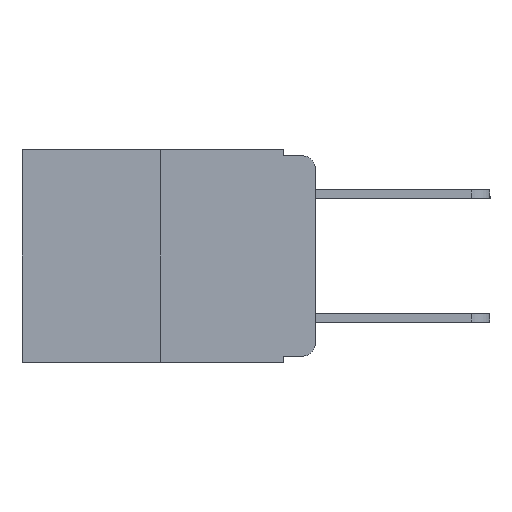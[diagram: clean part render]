
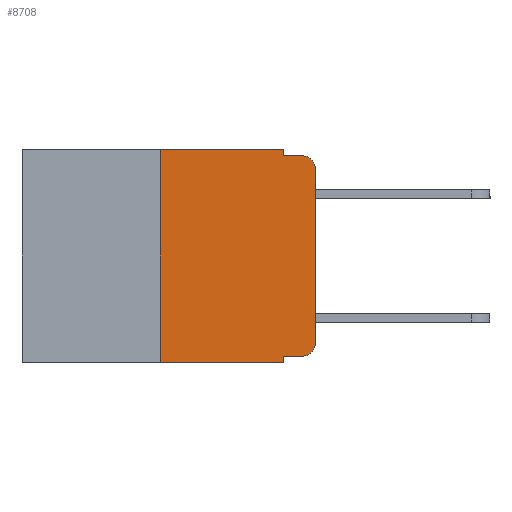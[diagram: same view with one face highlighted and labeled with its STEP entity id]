
A CAD part, left-side view. The second image highlights one B-rep face of the part: STEP entity #8708.
In plain terms, the highlighted planar face has unit normal (-1, 0, 0).
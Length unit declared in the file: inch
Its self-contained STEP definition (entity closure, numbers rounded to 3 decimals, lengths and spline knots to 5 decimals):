
#329 = ORIENTED_EDGE ( 'NONE', *, *, #9230, .F. ) ;
#381 = ORIENTED_EDGE ( 'NONE', *, *, #10804, .T. ) ;
#391 = ORIENTED_EDGE ( 'NONE', *, *, #2260, .F. ) ;
#1883 = CARTESIAN_POINT ( 'NONE',  ( 0., 0.051, -0.01 ) ) ;
#2018 = AXIS2_PLACEMENT_3D ( 'NONE', #16356, #8391, #11238 ) ;
#2258 = DIRECTION ( 'NONE',  ( 0., 0., 1. ) ) ;
#2260 = EDGE_CURVE ( 'NONE', #4453, #10729, #8984, .T. ) ;
#2508 = VERTEX_POINT ( 'NONE', #9882 ) ;
#2665 = CARTESIAN_POINT ( 'NONE',  ( 0., 0.02, -0.313 ) ) ;
#2958 = VECTOR ( 'NONE', #15019, 39.37008 ) ;
#3173 = CARTESIAN_POINT ( 'NONE',  ( 0., 0.051, 0. ) ) ;
#3475 = CARTESIAN_POINT ( 'NONE',  ( 0., 0.02, -0.01 ) ) ;
#3647 = VERTEX_POINT ( 'NONE', #17110 ) ;
#4095 = DIRECTION ( 'NONE',  ( 0., 0., 1. ) ) ;
#4104 = VECTOR ( 'NONE', #10636, 39.37008 ) ;
#4248 = VERTEX_POINT ( 'NONE', #4349 ) ;
#4349 = CARTESIAN_POINT ( 'NONE',  ( 0., 0.25, 0. ) ) ;
#4357 = DIRECTION ( 'NONE',  ( 0., 0., -1. ) ) ;
#4453 = VERTEX_POINT ( 'NONE', #7680 ) ;
#4612 = VERTEX_POINT ( 'NONE', #3475 ) ;
#4946 = LINE ( 'NONE', #14406, #8541 ) ;
#5039 = EDGE_LOOP ( 'NONE', ( #12263, #12685, #16614, #391, #329, #8214, #17254, #11268, #15150, #381 ) ) ;
#5049 = CARTESIAN_POINT ( 'NONE',  ( 0., 0.25, -0.343 ) ) ;
#5187 = VECTOR ( 'NONE', #15256, 39.37008 ) ;
#5480 = CARTESIAN_POINT ( 'NONE',  ( 0., 0.473, -0.343 ) ) ;
#5795 = EDGE_CURVE ( 'NONE', #2508, #3647, #15393, .T. ) ;
#5852 = VECTOR ( 'NONE', #11957, 39.37008 ) ;
#6026 = CARTESIAN_POINT ( 'NONE',  ( 0., 0.051, -0.333 ) ) ;
#7145 = LINE ( 'NONE', #1883, #2958 ) ;
#7378 = PLANE ( 'NONE',  #13105 ) ;
#7387 = EDGE_CURVE ( 'NONE', #15232, #4612, #9110, .T. ) ;
#7433 = CARTESIAN_POINT ( 'NONE',  ( 0., 0.473, 0. ) ) ;
#7680 = CARTESIAN_POINT ( 'NONE',  ( 0., 0.051, 0. ) ) ;
#7707 = LINE ( 'NONE', #3173, #8732 ) ;
#8214 = ORIENTED_EDGE ( 'NONE', *, *, #12314, .F. ) ;
#8391 = DIRECTION ( 'NONE',  ( -1., 0., 0. ) ) ;
#8541 = VECTOR ( 'NONE', #18064, 39.37008 ) ;
#8708 = ADVANCED_FACE ( 'NONE', ( #9063 ), #7378, .F. ) ;
#8732 = VECTOR ( 'NONE', #14728, 39.37008 ) ;
#8843 = VERTEX_POINT ( 'NONE', #17114 ) ;
#8913 = VECTOR ( 'NONE', #4095, 39.37008 ) ;
#8984 = LINE ( 'NONE', #11843, #5852 ) ;
#9034 = DIRECTION ( 'NONE',  ( 0., 0., -1. ) ) ;
#9063 = FACE_OUTER_BOUND ( 'NONE', #5039, .T. ) ;
#9110 = CIRCLE ( 'NONE', #2018, 0.02 ) ;
#9230 = EDGE_CURVE ( 'NONE', #4248, #4453, #4946, .T. ) ;
#9335 = LINE ( 'NONE', #11478, #8913 ) ;
#9690 = CARTESIAN_POINT ( 'NONE',  ( 0., 0.051, -0.343 ) ) ;
#9776 = LINE ( 'NONE', #11377, #16689 ) ;
#9882 = CARTESIAN_POINT ( 'NONE',  ( 0., 0.051, -0.333 ) ) ;
#10411 = VERTEX_POINT ( 'NONE', #5049 ) ;
#10636 = DIRECTION ( 'NONE',  ( 0., -1., 0. ) ) ;
#10729 = VERTEX_POINT ( 'NONE', #11518 ) ;
#10804 = EDGE_CURVE ( 'NONE', #3647, #8843, #18512, .T. ) ;
#11099 = EDGE_CURVE ( 'NONE', #2508, #16935, #7707, .T. ) ;
#11132 = AXIS2_PLACEMENT_3D ( 'NONE', #2665, #13030, #4357 ) ;
#11238 = DIRECTION ( 'NONE',  ( 0., 0., -1. ) ) ;
#11268 = ORIENTED_EDGE ( 'NONE', *, *, #11099, .F. ) ;
#11377 = CARTESIAN_POINT ( 'NONE',  ( 0., 0., 0. ) ) ;
#11478 = CARTESIAN_POINT ( 'NONE',  ( 0., 0.25, 0. ) ) ;
#11518 = CARTESIAN_POINT ( 'NONE',  ( 0., 0.051, -0.01 ) ) ;
#11843 = CARTESIAN_POINT ( 'NONE',  ( 0., 0.051, 0. ) ) ;
#11957 = DIRECTION ( 'NONE',  ( 0., 0., -1. ) ) ;
#11973 = CARTESIAN_POINT ( 'NONE',  ( 0., 0., -0.03 ) ) ;
#12210 = EDGE_CURVE ( 'NONE', #8843, #15232, #9776, .T. ) ;
#12263 = ORIENTED_EDGE ( 'NONE', *, *, #12210, .T. ) ;
#12314 = EDGE_CURVE ( 'NONE', #10411, #4248, #9335, .T. ) ;
#12685 = ORIENTED_EDGE ( 'NONE', *, *, #7387, .T. ) ;
#13030 = DIRECTION ( 'NONE',  ( -1., 0., 0. ) ) ;
#13105 = AXIS2_PLACEMENT_3D ( 'NONE', #7433, #16846, #9034 ) ;
#14406 = CARTESIAN_POINT ( 'NONE',  ( 0., 0.473, 0. ) ) ;
#14681 = EDGE_CURVE ( 'NONE', #10729, #4612, #7145, .T. ) ;
#14728 = DIRECTION ( 'NONE',  ( 0., 0., -1. ) ) ;
#15019 = DIRECTION ( 'NONE',  ( 0., -1., 0. ) ) ;
#15150 = ORIENTED_EDGE ( 'NONE', *, *, #5795, .T. ) ;
#15232 = VERTEX_POINT ( 'NONE', #11973 ) ;
#15256 = DIRECTION ( 'NONE',  ( 0., -1., 0. ) ) ;
#15393 = LINE ( 'NONE', #6026, #4104 ) ;
#15842 = LINE ( 'NONE', #5480, #5187 ) ;
#16356 = CARTESIAN_POINT ( 'NONE',  ( 0., 0.02, -0.03 ) ) ;
#16400 = EDGE_CURVE ( 'NONE', #10411, #16935, #15842, .T. ) ;
#16614 = ORIENTED_EDGE ( 'NONE', *, *, #14681, .F. ) ;
#16689 = VECTOR ( 'NONE', #2258, 39.37008 ) ;
#16846 = DIRECTION ( 'NONE',  ( 1., 0., 0. ) ) ;
#16935 = VERTEX_POINT ( 'NONE', #9690 ) ;
#17110 = CARTESIAN_POINT ( 'NONE',  ( 0., 0.02, -0.333 ) ) ;
#17114 = CARTESIAN_POINT ( 'NONE',  ( 0., 0., -0.313 ) ) ;
#17254 = ORIENTED_EDGE ( 'NONE', *, *, #16400, .T. ) ;
#18064 = DIRECTION ( 'NONE',  ( 0., -1., 0. ) ) ;
#18512 = CIRCLE ( 'NONE', #11132, 0.02 ) ;
